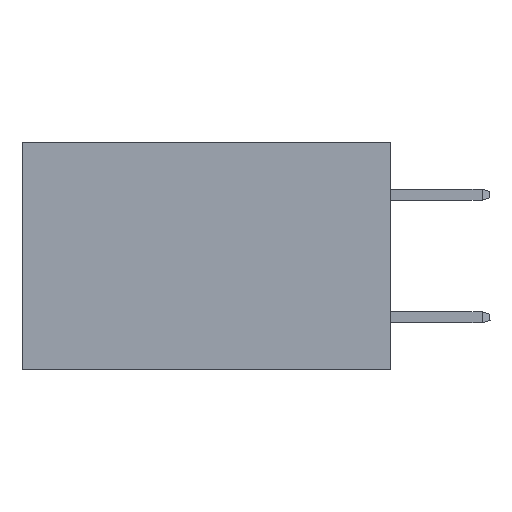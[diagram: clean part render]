
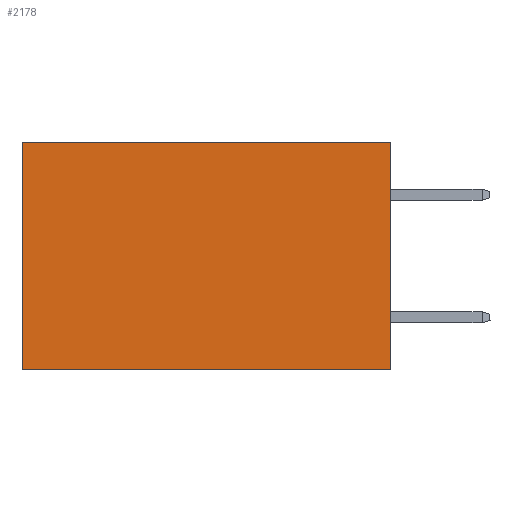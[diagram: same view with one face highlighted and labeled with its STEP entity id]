
A CAD part, left-side view. The second image highlights one B-rep face of the part: STEP entity #2178.
In plain terms, the highlighted planar face has unit normal (-1, 0, 0).
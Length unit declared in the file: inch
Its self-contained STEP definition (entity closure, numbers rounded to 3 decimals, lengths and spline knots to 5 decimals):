
#444 = VECTOR ( 'NONE', #11978, 39.37008 ) ;
#1459 = VERTEX_POINT ( 'NONE', #36654 ) ;
#2178 = ADVANCED_FACE ( 'NONE', ( #33788 ), #14997, .F. ) ;
#3158 = VECTOR ( 'NONE', #27255, 39.37008 ) ;
#3699 = CARTESIAN_POINT ( 'NONE',  ( 0.2875, 0.6, 0. ) ) ;
#4129 = ORIENTED_EDGE ( 'NONE', *, *, #35405, .T. ) ;
#7698 = LINE ( 'NONE', #33106, #3158 ) ;
#9437 = CARTESIAN_POINT ( 'NONE',  ( 0.2875, 0., 0. ) ) ;
#10420 = VERTEX_POINT ( 'NONE', #32767 ) ;
#11978 = DIRECTION ( 'NONE',  ( 0., 0., -1. ) ) ;
#12233 = DIRECTION ( 'NONE',  ( 1., 0., 0. ) ) ;
#12234 = CARTESIAN_POINT ( 'NONE',  ( 0.2875, 0., 0. ) ) ;
#13195 = ORIENTED_EDGE ( 'NONE', *, *, #16806, .F. ) ;
#13368 = VERTEX_POINT ( 'NONE', #16220 ) ;
#14094 = EDGE_CURVE ( 'NONE', #1459, #18013, #32003, .T. ) ;
#14997 = PLANE ( 'NONE',  #19467 ) ;
#16220 = CARTESIAN_POINT ( 'NONE',  ( 0.2875, 0., 0. ) ) ;
#16806 = EDGE_CURVE ( 'NONE', #13368, #1459, #25810, .T. ) ;
#16842 = EDGE_CURVE ( 'NONE', #13368, #10420, #7698, .T. ) ;
#17066 = EDGE_LOOP ( 'NONE', ( #4129, #24440, #13195, #18578 ) ) ;
#18013 = VERTEX_POINT ( 'NONE', #29534 ) ;
#18578 = ORIENTED_EDGE ( 'NONE', *, *, #16842, .T. ) ;
#19467 = AXIS2_PLACEMENT_3D ( 'NONE', #9437, #12233, #23436 ) ;
#20319 = VECTOR ( 'NONE', #27097, 39.37008 ) ;
#21230 = LINE ( 'NONE', #3699, #20319 ) ;
#23436 = DIRECTION ( 'NONE',  ( 0., 0., -1. ) ) ;
#24440 = ORIENTED_EDGE ( 'NONE', *, *, #14094, .F. ) ;
#25810 = LINE ( 'NONE', #12234, #444 ) ;
#27097 = DIRECTION ( 'NONE',  ( 0., 0., -1. ) ) ;
#27255 = DIRECTION ( 'NONE',  ( 0., 1., 0. ) ) ;
#29534 = CARTESIAN_POINT ( 'NONE',  ( 0.2875, 0.6, -0.37 ) ) ;
#29707 = CARTESIAN_POINT ( 'NONE',  ( 0.2875, 0., -0.37 ) ) ;
#32003 = LINE ( 'NONE', #29707, #36522 ) ;
#32185 = DIRECTION ( 'NONE',  ( 0., 1., 0. ) ) ;
#32767 = CARTESIAN_POINT ( 'NONE',  ( 0.2875, 0.6, 0. ) ) ;
#33106 = CARTESIAN_POINT ( 'NONE',  ( 0.2875, 0., 0. ) ) ;
#33788 = FACE_OUTER_BOUND ( 'NONE', #17066, .T. ) ;
#35405 = EDGE_CURVE ( 'NONE', #10420, #18013, #21230, .T. ) ;
#36522 = VECTOR ( 'NONE', #32185, 39.37008 ) ;
#36654 = CARTESIAN_POINT ( 'NONE',  ( 0.2875, 0., -0.37 ) ) ;
